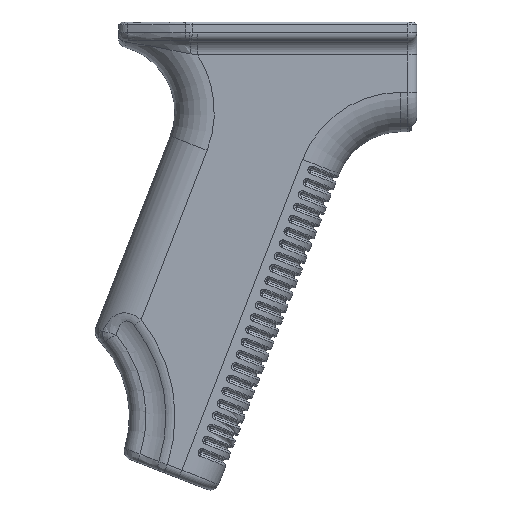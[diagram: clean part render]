
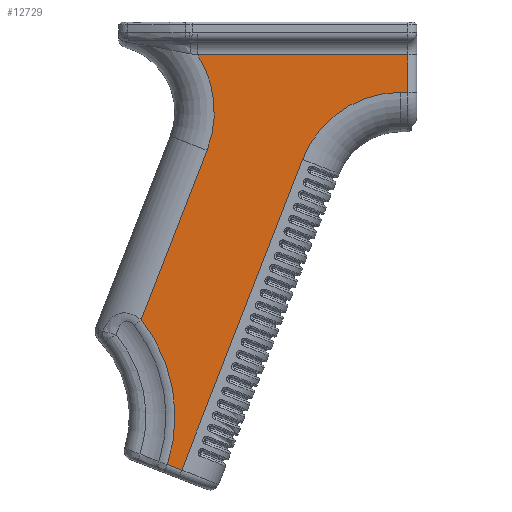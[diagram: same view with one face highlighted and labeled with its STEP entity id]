
A CAD part, front view. The second image highlights one B-rep face of the part: STEP entity #12729.
In plain terms, the highlighted planar face has unit normal (0, -1, 0).
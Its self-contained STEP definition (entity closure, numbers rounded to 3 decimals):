
#595=PLANE('',#14364);
#1397=FACE_OUTER_BOUND('',#2233,.T.);
#2233=EDGE_LOOP('',(#11537,#11538,#11539,#11540,#11541,#11542,#11543,#11544,
#11545));
#2714=LINE('',#19815,#3300);
#3037=LINE('',#26949,#3623);
#3041=LINE('',#27428,#3627);
#3108=LINE('',#28659,#3694);
#3115=LINE('',#28722,#3701);
#3122=LINE('',#28790,#3708);
#3300=VECTOR('',#14887,10.);
#3623=VECTOR('',#17398,10.);
#3627=VECTOR('',#17462,10.);
#3694=VECTOR('',#17701,10.);
#3701=VECTOR('',#17728,10.);
#3708=VECTOR('',#17761,10.);
#4604=CIRCLE('',#14081,35.365);
#4638=CIRCLE('',#14141,24.18);
#4752=CIRCLE('',#14365,24.);
#5037=VERTEX_POINT('',#19812);
#5038=VERTEX_POINT('',#19814);
#5594=VERTEX_POINT('',#26930);
#5596=VERTEX_POINT('',#26948);
#5608=VERTEX_POINT('',#27264);
#5648=VERTEX_POINT('',#27636);
#5742=VERTEX_POINT('',#28652);
#5744=VERTEX_POINT('',#28657);
#5753=VERTEX_POINT('',#28721);
#6195=EDGE_CURVE('',#5037,#5038,#2714,.T.);
#7293=EDGE_CURVE('',#5594,#5596,#3037,.T.);
#7321=EDGE_CURVE('',#5608,#5594,#4604,.T.);
#7336=EDGE_CURVE('',#5038,#5608,#3041,.T.);
#7393=EDGE_CURVE('',#5596,#5648,#4638,.T.);
#7522=EDGE_CURVE('',#5744,#5742,#3108,.T.);
#7537=EDGE_CURVE('',#5742,#5753,#3115,.T.);
#7555=EDGE_CURVE('',#5648,#5744,#3122,.T.);
#7775=EDGE_CURVE('',#5753,#5037,#4752,.T.);
#11537=ORIENTED_EDGE('',*,*,#7775,.F.);
#11538=ORIENTED_EDGE('',*,*,#7537,.F.);
#11539=ORIENTED_EDGE('',*,*,#7522,.F.);
#11540=ORIENTED_EDGE('',*,*,#7555,.F.);
#11541=ORIENTED_EDGE('',*,*,#7393,.F.);
#11542=ORIENTED_EDGE('',*,*,#7293,.F.);
#11543=ORIENTED_EDGE('',*,*,#7321,.F.);
#11544=ORIENTED_EDGE('',*,*,#7336,.F.);
#11545=ORIENTED_EDGE('',*,*,#6195,.F.);
#12729=ADVANCED_FACE('',(#1397),#595,.F.);
#14081=AXIS2_PLACEMENT_3D('',#27270,#17427,#17428);
#14141=AXIS2_PLACEMENT_3D('',#27637,#17572,#17573);
#14364=AXIS2_PLACEMENT_3D('',#30250,#18164,#18165);
#14365=AXIS2_PLACEMENT_3D('',#30251,#18166,#18167);
#14887=DIRECTION('',(-0.362,0.,-0.932));
#17398=DIRECTION('',(0.362,0.,0.932));
#17427=DIRECTION('center_axis',(0.,-1.,0.));
#17428=DIRECTION('ref_axis',(0.99,0.,0.14));
#17462=DIRECTION('',(-0.932,0.,0.362));
#17572=DIRECTION('center_axis',(0.,-1.,0.));
#17573=DIRECTION('ref_axis',(0.868,0.,0.497));
#17701=DIRECTION('',(0.,0.,-1.));
#17728=DIRECTION('',(-1.,0.,0.));
#17761=DIRECTION('',(1.,0.,0.));
#18164=DIRECTION('center_axis',(0.,1.,0.));
#18165=DIRECTION('ref_axis',(0.,0.,
1.));
#18166=DIRECTION('center_axis',(0.,-1.,0.));
#18167=DIRECTION('ref_axis',(-0.565,0.,0.825));
#19812=CARTESIAN_POINT('',(23.393,9.9,-31.301));
#19814=CARTESIAN_POINT('',(-4.104,9.9,-102.009));
#19815=CARTESIAN_POINT('',(-0.02,9.9,-91.506));
#26930=CARTESIAN_POINT('',(-13.327,9.9,-67.785));
#26948=CARTESIAN_POINT('',(1.667,9.9,-29.228));
#26949=CARTESIAN_POINT('',(-19.592,9.9,-83.895));
#27264=CARTESIAN_POINT('',(-7.366,9.9,-100.74));
#27270=CARTESIAN_POINT('Origin',(-40.999,9.9,-89.807));
#27428=CARTESIAN_POINT('',(-45.246,9.9,-86.009));
#27636=CARTESIAN_POINT('',(-0.458,9.9,-7.5));
#27637=CARTESIAN_POINT('Origin',(-20.869,9.9,-20.464));
#28652=CARTESIAN_POINT('',(47.401,9.9,-16.));
#28657=CARTESIAN_POINT('',(47.401,9.9,-7.5));
#28659=CARTESIAN_POINT('',(47.401,9.9,-85.346));
#28721=CARTESIAN_POINT('',(45.761,9.9,-16.));
#28722=CARTESIAN_POINT('',(-15.86,9.9,-16.));
#28790=CARTESIAN_POINT('',(9.41,9.9,-7.5));
#30250=CARTESIAN_POINT('Origin',(-30.38,9.9,-6.));
#30251=CARTESIAN_POINT('Origin',(45.761,9.9,-40.));
